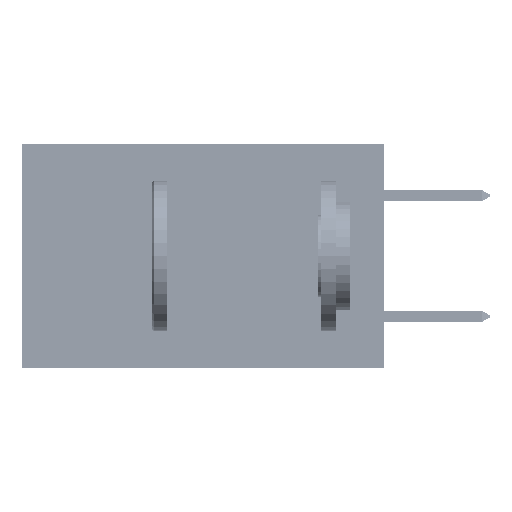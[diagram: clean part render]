
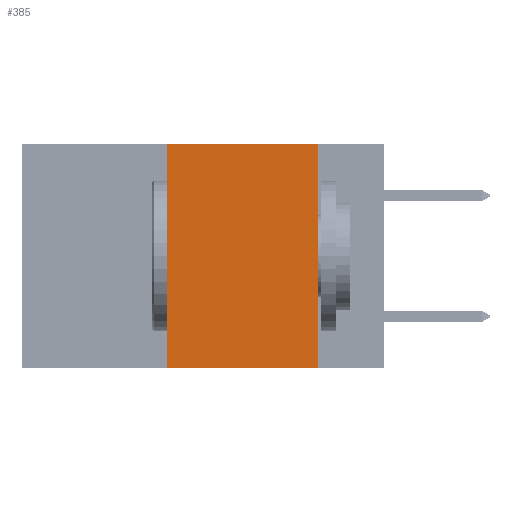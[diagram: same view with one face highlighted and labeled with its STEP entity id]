
A CAD part, left-side view. The second image highlights one B-rep face of the part: STEP entity #385.
In plain terms, the highlighted planar face has unit normal (-1, 0, 0).
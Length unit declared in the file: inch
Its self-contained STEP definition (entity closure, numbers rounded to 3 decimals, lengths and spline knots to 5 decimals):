
#40 = EDGE_CURVE ( 'NONE', #6790, #46142, #21416, .T. ) ;
#385 = ADVANCED_FACE ( 'NONE', ( #30962 ), #46803, .F. ) ;
#1295 = VECTOR ( 'NONE', #7630, 39.37008 ) ;
#4224 = VECTOR ( 'NONE', #10303, 39.37008 ) ;
#5810 = CARTESIAN_POINT ( 'NONE',  ( 0., 0.6, -0.37 ) ) ;
#6790 = VERTEX_POINT ( 'NONE', #37773 ) ;
#7630 = DIRECTION ( 'NONE',  ( 0., 0., 1. ) ) ;
#8016 = CARTESIAN_POINT ( 'NONE',  ( 0., 0.6, 0. ) ) ;
#8022 = ORIENTED_EDGE ( 'NONE', *, *, #40, .F. ) ;
#9209 = EDGE_CURVE ( 'NONE', #35451, #6790, #31948, .T. ) ;
#10303 = DIRECTION ( 'NONE',  ( 0., -1., 0. ) ) ;
#11182 = ORIENTED_EDGE ( 'NONE', *, *, #13954, .T. ) ;
#13536 = LINE ( 'NONE', #19946, #1295 ) ;
#13954 = EDGE_CURVE ( 'NONE', #14067, #46142, #36535, .T. ) ;
#14067 = VERTEX_POINT ( 'NONE', #31759 ) ;
#14147 = CARTESIAN_POINT ( 'NONE',  ( 0., 0.6, 0. ) ) ;
#15161 = VECTOR ( 'NONE', #38379, 39.37008 ) ;
#17477 = EDGE_CURVE ( 'NONE', #14067, #35451, #13536, .T. ) ;
#17597 = DIRECTION ( 'NONE',  ( 0., 0., -1. ) ) ;
#18486 = CARTESIAN_POINT ( 'NONE',  ( 0., 0.36, 0. ) ) ;
#19946 = CARTESIAN_POINT ( 'NONE',  ( 0., 0.36, 0. ) ) ;
#21416 = LINE ( 'NONE', #30650, #29065 ) ;
#27819 = AXIS2_PLACEMENT_3D ( 'NONE', #14147, #47159, #17597 ) ;
#29065 = VECTOR ( 'NONE', #38839, 39.37008 ) ;
#30650 = CARTESIAN_POINT ( 'NONE',  ( 0., 0.11, 0. ) ) ;
#30962 = FACE_OUTER_BOUND ( 'NONE', #44585, .T. ) ;
#31759 = CARTESIAN_POINT ( 'NONE',  ( 0., 0.36, -0.37 ) ) ;
#31948 = LINE ( 'NONE', #8016, #15161 ) ;
#35451 = VERTEX_POINT ( 'NONE', #18486 ) ;
#36535 = LINE ( 'NONE', #5810, #4224 ) ;
#37521 = ORIENTED_EDGE ( 'NONE', *, *, #9209, .F. ) ;
#37773 = CARTESIAN_POINT ( 'NONE',  ( 0., 0.11, 0. ) ) ;
#38379 = DIRECTION ( 'NONE',  ( 0., -1., 0. ) ) ;
#38839 = DIRECTION ( 'NONE',  ( 0., 0., -1. ) ) ;
#39153 = CARTESIAN_POINT ( 'NONE',  ( 0., 0.11, -0.37 ) ) ;
#39240 = ORIENTED_EDGE ( 'NONE', *, *, #17477, .F. ) ;
#44585 = EDGE_LOOP ( 'NONE', ( #8022, #37521, #39240, #11182 ) ) ;
#46142 = VERTEX_POINT ( 'NONE', #39153 ) ;
#46803 = PLANE ( 'NONE',  #27819 ) ;
#47159 = DIRECTION ( 'NONE',  ( 1., 0., 0. ) ) ;
